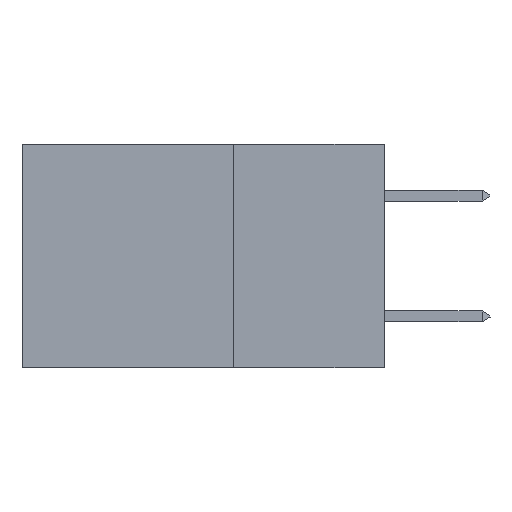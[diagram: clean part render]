
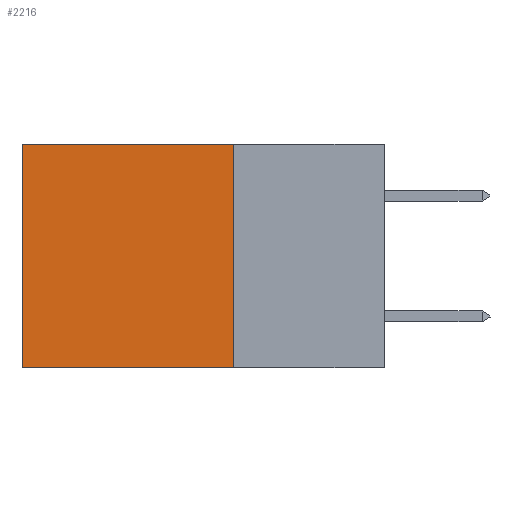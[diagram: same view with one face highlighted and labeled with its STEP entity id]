
A CAD part, left-side view. The second image highlights one B-rep face of the part: STEP entity #2216.
In plain terms, the highlighted planar face has unit normal (-1, 0, 0).
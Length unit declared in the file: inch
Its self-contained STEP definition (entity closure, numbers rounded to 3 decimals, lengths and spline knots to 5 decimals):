
#207 = VECTOR ( 'NONE', #5471, 39.37008 ) ;
#922 = CARTESIAN_POINT ( 'NONE',  ( 0.2875, 0.25, -0.37 ) ) ;
#968 = CARTESIAN_POINT ( 'NONE',  ( 0.2875, 0.25, 0. ) ) ;
#1306 = LINE ( 'NONE', #1758, #207 ) ;
#1427 = AXIS2_PLACEMENT_3D ( 'NONE', #5775, #9229, #2024 ) ;
#1758 = CARTESIAN_POINT ( 'NONE',  ( 0.2875, 0.6, 0. ) ) ;
#2024 = DIRECTION ( 'NONE',  ( 0., 0., -1. ) ) ;
#2216 = ADVANCED_FACE ( 'NONE', ( #7867 ), #9336, .F. ) ;
#3502 = VECTOR ( 'NONE', #4834, 39.37008 ) ;
#3539 = VECTOR ( 'NONE', #4559, 39.37008 ) ;
#3577 = EDGE_LOOP ( 'NONE', ( #10439, #11443, #6219, #9927 ) ) ;
#4559 = DIRECTION ( 'NONE',  ( 0., 0., -1. ) ) ;
#4834 = DIRECTION ( 'NONE',  ( 0., 1., 0. ) ) ;
#4976 = EDGE_CURVE ( 'NONE', #11040, #9313, #9068, .T. ) ;
#5310 = EDGE_CURVE ( 'NONE', #11544, #6851, #1306, .T. ) ;
#5471 = DIRECTION ( 'NONE',  ( 0., 0., -1. ) ) ;
#5584 = LINE ( 'NONE', #10721, #9932 ) ;
#5775 = CARTESIAN_POINT ( 'NONE',  ( 0.2875, 0.25, 0. ) ) ;
#6219 = ORIENTED_EDGE ( 'NONE', *, *, #4976, .F. ) ;
#6236 = LINE ( 'NONE', #9438, #3502 ) ;
#6481 = EDGE_CURVE ( 'NONE', #11040, #11544, #6236, .T. ) ;
#6762 = CARTESIAN_POINT ( 'NONE',  ( 0.2875, 0.6, 0. ) ) ;
#6851 = VERTEX_POINT ( 'NONE', #7352 ) ;
#7352 = CARTESIAN_POINT ( 'NONE',  ( 0.2875, 0.6, -0.37 ) ) ;
#7867 = FACE_OUTER_BOUND ( 'NONE', #3577, .T. ) ;
#8190 = DIRECTION ( 'NONE',  ( 0., 1., 0. ) ) ;
#8729 = CARTESIAN_POINT ( 'NONE',  ( 0.2875, 0.25, 0. ) ) ;
#9068 = LINE ( 'NONE', #968, #3539 ) ;
#9229 = DIRECTION ( 'NONE',  ( 1., 0., 0. ) ) ;
#9313 = VERTEX_POINT ( 'NONE', #922 ) ;
#9336 = PLANE ( 'NONE',  #1427 ) ;
#9438 = CARTESIAN_POINT ( 'NONE',  ( 0.2875, 0.25, 0. ) ) ;
#9927 = ORIENTED_EDGE ( 'NONE', *, *, #6481, .T. ) ;
#9932 = VECTOR ( 'NONE', #8190, 39.37008 ) ;
#10019 = EDGE_CURVE ( 'NONE', #9313, #6851, #5584, .T. ) ;
#10439 = ORIENTED_EDGE ( 'NONE', *, *, #5310, .T. ) ;
#10721 = CARTESIAN_POINT ( 'NONE',  ( 0.2875, 0.25, -0.37 ) ) ;
#11040 = VERTEX_POINT ( 'NONE', #8729 ) ;
#11443 = ORIENTED_EDGE ( 'NONE', *, *, #10019, .F. ) ;
#11544 = VERTEX_POINT ( 'NONE', #6762 ) ;
